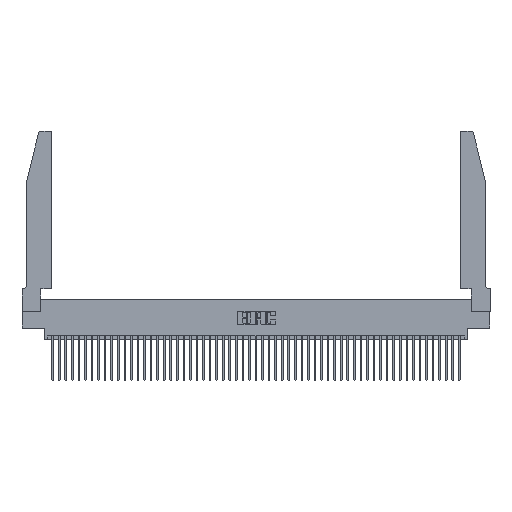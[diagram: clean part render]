
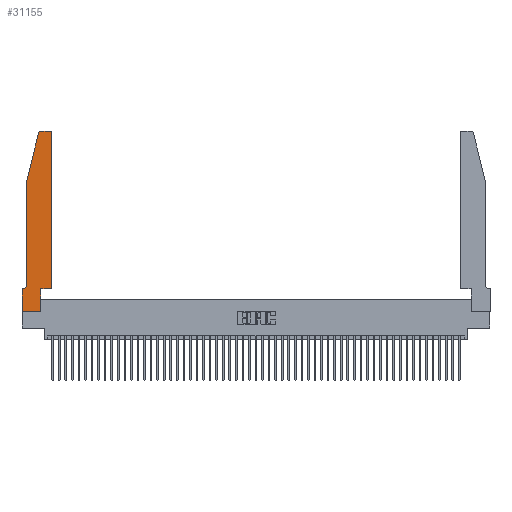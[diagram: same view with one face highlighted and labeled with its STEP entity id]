
A CAD part, top view. The second image highlights one B-rep face of the part: STEP entity #31155.
In plain terms, the highlighted planar face has unit normal (0, 0, 1).
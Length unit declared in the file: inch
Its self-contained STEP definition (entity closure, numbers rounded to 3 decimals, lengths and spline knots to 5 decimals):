
#1072 = CARTESIAN_POINT ( 'NONE',  ( 0.284, 2.75, 0.37 ) ) ;
#1295 = DIRECTION ( 'NONE',  ( 0., 1., 0. ) ) ;
#1522 = DIRECTION ( 'NONE',  ( 0., 0., 1. ) ) ;
#1709 = DIRECTION ( 'NONE',  ( -1., 0., 0. ) ) ;
#1975 = CARTESIAN_POINT ( 'NONE',  ( 0.4505, 0.35, 0.37 ) ) ;
#2455 = CARTESIAN_POINT ( 'NONE',  ( 0.2865, 0.35, 0.37 ) ) ;
#2627 = CARTESIAN_POINT ( 'NONE',  ( 0.2605, 2.75, 0.37 ) ) ;
#2975 = CARTESIAN_POINT ( 'NONE',  ( 0., 0., 0.37 ) ) ;
#3922 = CARTESIAN_POINT ( 'NONE',  ( 0.0055, 0.42, 0.37 ) ) ;
#4667 = CIRCLE ( 'NONE', #21103, 0.03 ) ;
#4862 = DIRECTION ( 'NONE',  ( 1., 0., 0. ) ) ;
#5177 = EDGE_CURVE ( 'NONE', #33209, #35162, #31062, .T. ) ;
#5384 = PLANE ( 'NONE',  #40700 ) ;
#5719 = CARTESIAN_POINT ( 'NONE',  ( 0.0755, 0.35, 0.37 ) ) ;
#6937 = ORIENTED_EDGE ( 'NONE', *, *, #24975, .T. ) ;
#7658 = ORIENTED_EDGE ( 'NONE', *, *, #11758, .T. ) ;
#7774 = DIRECTION ( 'NONE',  ( -1., 0., 0. ) ) ;
#8127 = EDGE_CURVE ( 'NONE', #30535, #50190, #8965, .T. ) ;
#8233 = VERTEX_POINT ( 'NONE', #18893 ) ;
#8965 = CIRCLE ( 'NONE', #10482, 0.03 ) ;
#9399 = ORIENTED_EDGE ( 'NONE', *, *, #9874, .T. ) ;
#9463 = VECTOR ( 'NONE', #42160, 39.37008 ) ;
#9874 = EDGE_CURVE ( 'NONE', #31177, #14811, #50316, .T. ) ;
#10132 = DIRECTION ( 'NONE',  ( 0., 0., 1. ) ) ;
#10482 = AXIS2_PLACEMENT_3D ( 'NONE', #45933, #10132, #41972 ) ;
#11758 = EDGE_CURVE ( 'NONE', #19635, #29021, #25893, .T. ) ;
#12055 = DIRECTION ( 'NONE',  ( 0., 0., 1. ) ) ;
#12363 = EDGE_CURVE ( 'NONE', #32869, #33209, #15956, .T. ) ;
#12847 = DIRECTION ( 'NONE',  ( 0., 1., 0. ) ) ;
#13095 = DIRECTION ( 'NONE',  ( 1., 0., 0. ) ) ;
#14198 = EDGE_CURVE ( 'NONE', #45328, #20907, #21400, .T. ) ;
#14502 = ORIENTED_EDGE ( 'NONE', *, *, #5177, .T. ) ;
#14811 = VERTEX_POINT ( 'NONE', #49515 ) ;
#15708 = CARTESIAN_POINT ( 'NONE',  ( 0.0755, 2., 0.37 ) ) ;
#15956 = LINE ( 'NONE', #29292, #20953 ) ;
#16862 = CARTESIAN_POINT ( 'NONE',  ( 0.4505, 0.35, 0.37 ) ) ;
#17208 = DIRECTION ( 'NONE',  ( 0., -1., 0. ) ) ;
#18893 = CARTESIAN_POINT ( 'NONE',  ( 0.4205, 2.75, 0.37 ) ) ;
#19469 = FACE_OUTER_BOUND ( 'NONE', #50084, .T. ) ;
#19544 = ORIENTED_EDGE ( 'NONE', *, *, #45437, .T. ) ;
#19635 = VERTEX_POINT ( 'NONE', #1975 ) ;
#20896 = EDGE_CURVE ( 'NONE', #20907, #32869, #49891, .T. ) ;
#20907 = VERTEX_POINT ( 'NONE', #45511 ) ;
#20953 = VECTOR ( 'NONE', #45906, 39.37008 ) ;
#21051 = CARTESIAN_POINT ( 'NONE',  ( 0.0755, 2., 0.37 ) ) ;
#21103 = AXIS2_PLACEMENT_3D ( 'NONE', #36905, #1522, #13095 ) ;
#21400 = LINE ( 'NONE', #5719, #25702 ) ;
#21436 = CARTESIAN_POINT ( 'NONE',  ( 0.4505, 0.35, 0.37 ) ) ;
#23720 = DIRECTION ( 'NONE',  ( -0.239, -0.971, 0. ) ) ;
#23767 = EDGE_CURVE ( 'NONE', #35162, #19635, #30951, .T. ) ;
#24093 = AXIS2_PLACEMENT_3D ( 'NONE', #3922, #31654, #7774 ) ;
#24398 = CIRCLE ( 'NONE', #24093, 0.07 ) ;
#24975 = EDGE_CURVE ( 'NONE', #29021, #8233, #4667, .T. ) ;
#25702 = VECTOR ( 'NONE', #1709, 39.37008 ) ;
#25893 = LINE ( 'NONE', #16862, #49503 ) ;
#26304 = LINE ( 'NONE', #2627, #9463 ) ;
#27800 = VECTOR ( 'NONE', #23720, 39.37008 ) ;
#28813 = VECTOR ( 'NONE', #34098, 39.37008 ) ;
#28943 = CARTESIAN_POINT ( 'NONE',  ( 0.25487, 2.72718, 0.37 ) ) ;
#29021 = VERTEX_POINT ( 'NONE', #29402 ) ;
#29292 = CARTESIAN_POINT ( 'NONE',  ( 0., 0., 0.37 ) ) ;
#29402 = CARTESIAN_POINT ( 'NONE',  ( 0.4505, 2.72, 0.37 ) ) ;
#29783 = VECTOR ( 'NONE', #1295, 39.37008 ) ;
#30535 = VERTEX_POINT ( 'NONE', #1072 ) ;
#30951 = LINE ( 'NONE', #21436, #32833 ) ;
#31062 = LINE ( 'NONE', #32696, #29783 ) ;
#31155 = ADVANCED_FACE ( 'NONE', ( #19469 ), #5384, .T. ) ;
#31177 = VERTEX_POINT ( 'NONE', #36914 ) ;
#31654 = DIRECTION ( 'NONE',  ( 0., 0., -1. ) ) ;
#32696 = CARTESIAN_POINT ( 'NONE',  ( 0.2865, 0.35, 0.37 ) ) ;
#32833 = VECTOR ( 'NONE', #44674, 39.37008 ) ;
#32869 = VERTEX_POINT ( 'NONE', #2975 ) ;
#33209 = VERTEX_POINT ( 'NONE', #44332 ) ;
#34098 = DIRECTION ( 'NONE',  ( 0., -1., 0. ) ) ;
#35012 = ORIENTED_EDGE ( 'NONE', *, *, #49784, .T. ) ;
#35162 = VERTEX_POINT ( 'NONE', #2455 ) ;
#36905 = CARTESIAN_POINT ( 'NONE',  ( 0.4205, 2.72, 0.37 ) ) ;
#36914 = CARTESIAN_POINT ( 'NONE',  ( 0.0755, 2., 0.37 ) ) ;
#37874 = LINE ( 'NONE', #15708, #27800 ) ;
#39701 = ORIENTED_EDGE ( 'NONE', *, *, #48104, .T. ) ;
#40037 = ORIENTED_EDGE ( 'NONE', *, *, #8127, .T. ) ;
#40700 = AXIS2_PLACEMENT_3D ( 'NONE', #47814, #12055, #4862 ) ;
#41906 = CARTESIAN_POINT ( 'NONE',  ( 0., 0., 0.37 ) ) ;
#41972 = DIRECTION ( 'NONE',  ( 1., 0., 0. ) ) ;
#42160 = DIRECTION ( 'NONE',  ( -1., 0., 0. ) ) ;
#42256 = VECTOR ( 'NONE', #17208, 39.37008 ) ;
#42373 = ORIENTED_EDGE ( 'NONE', *, *, #12363, .T. ) ;
#44332 = CARTESIAN_POINT ( 'NONE',  ( 0.2865, 0., 0.37 ) ) ;
#44674 = DIRECTION ( 'NONE',  ( 1., 0., 0. ) ) ;
#45328 = VERTEX_POINT ( 'NONE', #47471 ) ;
#45437 = EDGE_CURVE ( 'NONE', #50190, #31177, #37874, .T. ) ;
#45511 = CARTESIAN_POINT ( 'NONE',  ( 0., 0.35, 0.37 ) ) ;
#45906 = DIRECTION ( 'NONE',  ( 1., 0., 0. ) ) ;
#45933 = CARTESIAN_POINT ( 'NONE',  ( 0.284, 2.72, 0.37 ) ) ;
#46893 = ORIENTED_EDGE ( 'NONE', *, *, #20896, .T. ) ;
#47023 = ORIENTED_EDGE ( 'NONE', *, *, #23767, .T. ) ;
#47471 = CARTESIAN_POINT ( 'NONE',  ( 0.0055, 0.35, 0.37 ) ) ;
#47814 = CARTESIAN_POINT ( 'NONE',  ( 0., 0.35, 0.37 ) ) ;
#48104 = EDGE_CURVE ( 'NONE', #14811, #45328, #24398, .T. ) ;
#49503 = VECTOR ( 'NONE', #12847, 39.37008 ) ;
#49515 = CARTESIAN_POINT ( 'NONE',  ( 0.0755, 0.42, 0.37 ) ) ;
#49784 = EDGE_CURVE ( 'NONE', #8233, #30535, #26304, .T. ) ;
#49891 = LINE ( 'NONE', #41906, #28813 ) ;
#50084 = EDGE_LOOP ( 'NONE', ( #35012, #40037, #19544, #9399, #39701, #50515, #46893, #42373, #14502, #47023, #7658, #6937 ) ) ;
#50190 = VERTEX_POINT ( 'NONE', #28943 ) ;
#50316 = LINE ( 'NONE', #21051, #42256 ) ;
#50515 = ORIENTED_EDGE ( 'NONE', *, *, #14198, .T. ) ;
